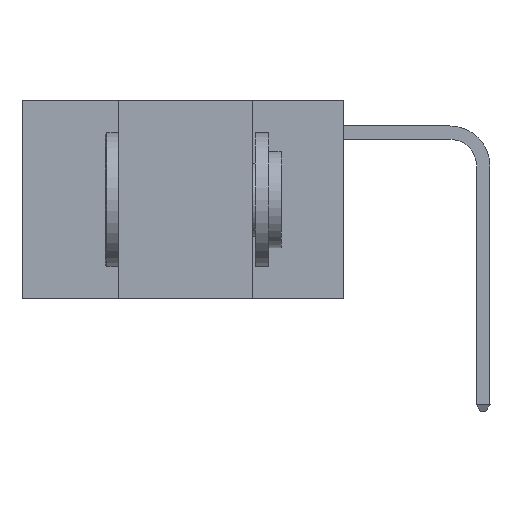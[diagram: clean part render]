
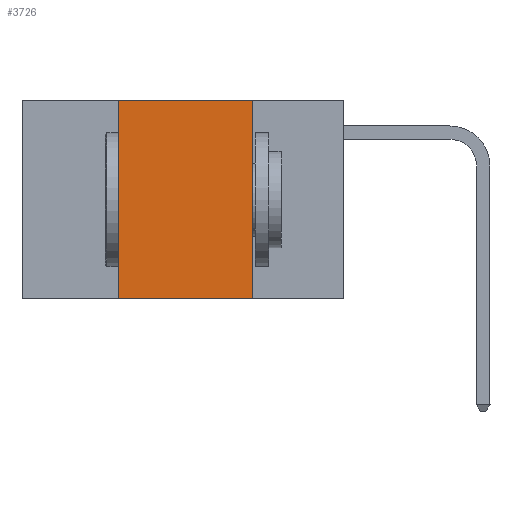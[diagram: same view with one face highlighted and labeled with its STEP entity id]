
A CAD part, left-side view. The second image highlights one B-rep face of the part: STEP entity #3726.
In plain terms, the highlighted planar face has unit normal (-1, 0, 0).
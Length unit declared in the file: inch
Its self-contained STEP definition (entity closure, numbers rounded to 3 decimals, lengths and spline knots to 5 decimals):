
#24 = DIRECTION ( 'NONE',  ( 1., 0., 0. ) ) ;
#261 = ORIENTED_EDGE ( 'NONE', *, *, #5612, .F. ) ;
#356 = VERTEX_POINT ( 'NONE', #6265 ) ;
#940 = LINE ( 'NONE', #1574, #2985 ) ;
#1282 = DIRECTION ( 'NONE',  ( 0., 0., -1. ) ) ;
#1523 = ORIENTED_EDGE ( 'NONE', *, *, #8900, .T. ) ;
#1574 = CARTESIAN_POINT ( 'NONE',  ( 0., 0.6, 0. ) ) ;
#1853 = VERTEX_POINT ( 'NONE', #8213 ) ;
#1879 = VERTEX_POINT ( 'NONE', #3417 ) ;
#2713 = ORIENTED_EDGE ( 'NONE', *, *, #9632, .F. ) ;
#2956 = DIRECTION ( 'NONE',  ( 0., 0., 1. ) ) ;
#2985 = VECTOR ( 'NONE', #8025, 39.37008 ) ;
#3298 = EDGE_CURVE ( 'NONE', #1853, #356, #9317, .T. ) ;
#3334 = LINE ( 'NONE', #5835, #3476 ) ;
#3417 = CARTESIAN_POINT ( 'NONE',  ( 0., 0.42, -0.37 ) ) ;
#3476 = VECTOR ( 'NONE', #4940, 39.37008 ) ;
#3605 = EDGE_LOOP ( 'NONE', ( #7489, #261, #2713, #1523 ) ) ;
#3726 = ADVANCED_FACE ( 'NONE', ( #6655 ), #7094, .F. ) ;
#3811 = CARTESIAN_POINT ( 'NONE',  ( 0., 0.42, 0. ) ) ;
#3920 = CARTESIAN_POINT ( 'NONE',  ( 0., 0.6, 0. ) ) ;
#4526 = CARTESIAN_POINT ( 'NONE',  ( 0., 0.17, 0. ) ) ;
#4867 = DIRECTION ( 'NONE',  ( 0., 0., -1. ) ) ;
#4940 = DIRECTION ( 'NONE',  ( 0., -1., 0. ) ) ;
#5483 = VECTOR ( 'NONE', #2956, 39.37008 ) ;
#5612 = EDGE_CURVE ( 'NONE', #7088, #1853, #940, .T. ) ;
#5835 = CARTESIAN_POINT ( 'NONE',  ( 0., 0.6, -0.37 ) ) ;
#6265 = CARTESIAN_POINT ( 'NONE',  ( 0., 0.17, -0.37 ) ) ;
#6632 = AXIS2_PLACEMENT_3D ( 'NONE', #3920, #24, #4867 ) ;
#6655 = FACE_OUTER_BOUND ( 'NONE', #3605, .T. ) ;
#7088 = VERTEX_POINT ( 'NONE', #3811 ) ;
#7094 = PLANE ( 'NONE',  #6632 ) ;
#7287 = CARTESIAN_POINT ( 'NONE',  ( 0., 0.42, 0. ) ) ;
#7489 = ORIENTED_EDGE ( 'NONE', *, *, #3298, .F. ) ;
#8025 = DIRECTION ( 'NONE',  ( 0., -1., 0. ) ) ;
#8213 = CARTESIAN_POINT ( 'NONE',  ( 0., 0.17, 0. ) ) ;
#8243 = VECTOR ( 'NONE', #1282, 39.37008 ) ;
#8900 = EDGE_CURVE ( 'NONE', #1879, #356, #3334, .T. ) ;
#9317 = LINE ( 'NONE', #4526, #8243 ) ;
#9412 = LINE ( 'NONE', #7287, #5483 ) ;
#9632 = EDGE_CURVE ( 'NONE', #1879, #7088, #9412, .T. ) ;
